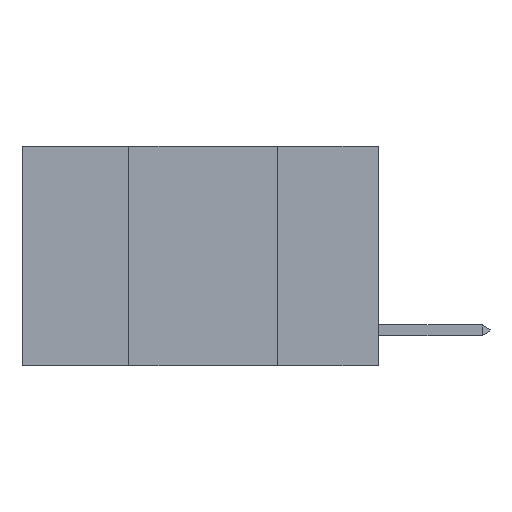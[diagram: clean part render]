
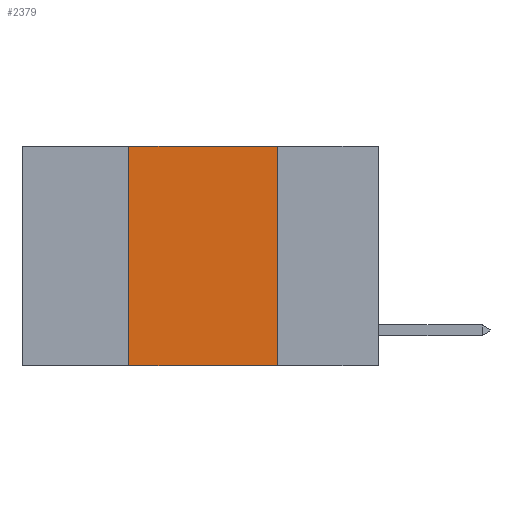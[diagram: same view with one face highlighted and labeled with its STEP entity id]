
A CAD part, left-side view. The second image highlights one B-rep face of the part: STEP entity #2379.
In plain terms, the highlighted planar face has unit normal (-1, 0, 0).
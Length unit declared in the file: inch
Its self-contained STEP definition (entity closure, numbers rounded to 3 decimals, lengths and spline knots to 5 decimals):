
#82 = ORIENTED_EDGE ( 'NONE', *, *, #6027, .F. ) ;
#701 = DIRECTION ( 'NONE',  ( 0., 0., -1. ) ) ;
#734 = FACE_OUTER_BOUND ( 'NONE', #5393, .T. ) ;
#1213 = CARTESIAN_POINT ( 'NONE',  ( 0., 0.6, 0. ) ) ;
#1279 = DIRECTION ( 'NONE',  ( 0., 0., 1. ) ) ;
#1624 = VERTEX_POINT ( 'NONE', #3796 ) ;
#2127 = LINE ( 'NONE', #8836, #4211 ) ;
#2203 = DIRECTION ( 'NONE',  ( 1., 0., 0. ) ) ;
#2379 = ADVANCED_FACE ( 'NONE', ( #734 ), #4932, .F. ) ;
#3211 = EDGE_CURVE ( 'NONE', #6827, #3486, #3532, .T. ) ;
#3457 = ORIENTED_EDGE ( 'NONE', *, *, #6663, .F. ) ;
#3486 = VERTEX_POINT ( 'NONE', #7254 ) ;
#3532 = LINE ( 'NONE', #4260, #7072 ) ;
#3796 = CARTESIAN_POINT ( 'NONE',  ( 0., 0.17, 0. ) ) ;
#4050 = CARTESIAN_POINT ( 'NONE',  ( 0., 0.17, -0.37 ) ) ;
#4211 = VECTOR ( 'NONE', #701, 39.37008 ) ;
#4260 = CARTESIAN_POINT ( 'NONE',  ( 0., 0.42, 0. ) ) ;
#4932 = PLANE ( 'NONE',  #4956 ) ;
#4956 = AXIS2_PLACEMENT_3D ( 'NONE', #6274, #2203, #6935 ) ;
#5362 = LINE ( 'NONE', #6270, #5780 ) ;
#5393 = EDGE_LOOP ( 'NONE', ( #82, #3457, #7829, #8539 ) ) ;
#5780 = VECTOR ( 'NONE', #6931, 39.37008 ) ;
#6027 = EDGE_CURVE ( 'NONE', #1624, #7343, #2127, .T. ) ;
#6077 = EDGE_CURVE ( 'NONE', #6827, #7343, #5362, .T. ) ;
#6270 = CARTESIAN_POINT ( 'NONE',  ( 0., 0.6, -0.37 ) ) ;
#6274 = CARTESIAN_POINT ( 'NONE',  ( 0., 0.6, 0. ) ) ;
#6663 = EDGE_CURVE ( 'NONE', #3486, #1624, #6883, .T. ) ;
#6827 = VERTEX_POINT ( 'NONE', #8769 ) ;
#6883 = LINE ( 'NONE', #1213, #8411 ) ;
#6931 = DIRECTION ( 'NONE',  ( 0., -1., 0. ) ) ;
#6935 = DIRECTION ( 'NONE',  ( 0., 0., -1. ) ) ;
#7072 = VECTOR ( 'NONE', #1279, 39.37008 ) ;
#7254 = CARTESIAN_POINT ( 'NONE',  ( 0., 0.42, 0. ) ) ;
#7343 = VERTEX_POINT ( 'NONE', #4050 ) ;
#7357 = DIRECTION ( 'NONE',  ( 0., -1., 0. ) ) ;
#7829 = ORIENTED_EDGE ( 'NONE', *, *, #3211, .F. ) ;
#8411 = VECTOR ( 'NONE', #7357, 39.37008 ) ;
#8539 = ORIENTED_EDGE ( 'NONE', *, *, #6077, .T. ) ;
#8769 = CARTESIAN_POINT ( 'NONE',  ( 0., 0.42, -0.37 ) ) ;
#8836 = CARTESIAN_POINT ( 'NONE',  ( 0., 0.17, 0. ) ) ;
